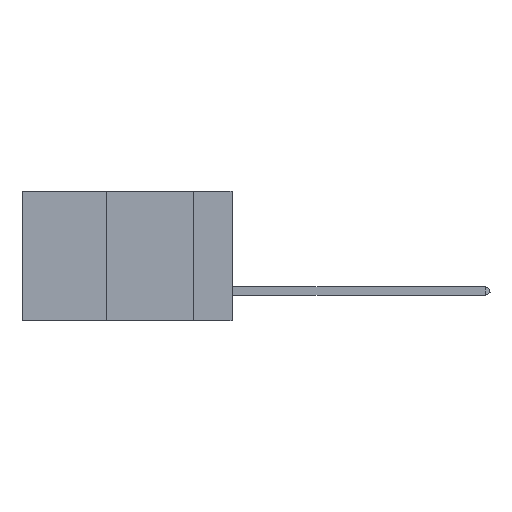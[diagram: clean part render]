
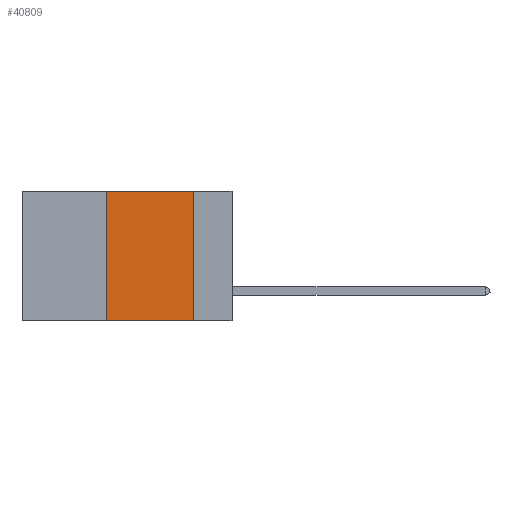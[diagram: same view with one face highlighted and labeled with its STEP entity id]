
A CAD part, left-side view. The second image highlights one B-rep face of the part: STEP entity #40809.
In plain terms, the highlighted planar face has unit normal (-1, 0, 0).
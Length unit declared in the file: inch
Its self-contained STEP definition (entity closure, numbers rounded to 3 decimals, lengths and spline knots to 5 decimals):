
#551 = DIRECTION ( 'NONE',  ( 0., -1., 0. ) ) ;
#1785 = VECTOR ( 'NONE', #551, 39.37008 ) ;
#2570 = EDGE_CURVE ( 'NONE', #17723, #35782, #29500, .T. ) ;
#2964 = VECTOR ( 'NONE', #40198, 39.37008 ) ;
#3206 = LINE ( 'NONE', #25588, #14075 ) ;
#4527 = ORIENTED_EDGE ( 'NONE', *, *, #42694, .F. ) ;
#5958 = FACE_OUTER_BOUND ( 'NONE', #35866, .T. ) ;
#7926 = PLANE ( 'NONE',  #23742 ) ;
#8074 = DIRECTION ( 'NONE',  ( 0., 0., -1. ) ) ;
#8186 = VECTOR ( 'NONE', #39829, 39.37008 ) ;
#10314 = CARTESIAN_POINT ( 'NONE',  ( 0., 0.11, -0.37 ) ) ;
#10552 = LINE ( 'NONE', #36775, #1785 ) ;
#14075 = VECTOR ( 'NONE', #31936, 39.37008 ) ;
#17723 = VERTEX_POINT ( 'NONE', #24574 ) ;
#19041 = LINE ( 'NONE', #20052, #2964 ) ;
#20052 = CARTESIAN_POINT ( 'NONE',  ( 0., 0.11, 0. ) ) ;
#20789 = DIRECTION ( 'NONE',  ( 1., 0., 0. ) ) ;
#21917 = EDGE_CURVE ( 'NONE', #35782, #30737, #10552, .T. ) ;
#21970 = VERTEX_POINT ( 'NONE', #10314 ) ;
#22845 = EDGE_CURVE ( 'NONE', #17723, #21970, #3206, .T. ) ;
#23742 = AXIS2_PLACEMENT_3D ( 'NONE', #24183, #20789, #8074 ) ;
#24183 = CARTESIAN_POINT ( 'NONE',  ( 0., 0.6, 0. ) ) ;
#24574 = CARTESIAN_POINT ( 'NONE',  ( 0., 0.36, -0.37 ) ) ;
#25588 = CARTESIAN_POINT ( 'NONE',  ( 0., 0.6, -0.37 ) ) ;
#26055 = CARTESIAN_POINT ( 'NONE',  ( 0., 0.11, 0. ) ) ;
#28347 = ORIENTED_EDGE ( 'NONE', *, *, #21917, .F. ) ;
#29495 = CARTESIAN_POINT ( 'NONE',  ( 0., 0.36, 0. ) ) ;
#29500 = LINE ( 'NONE', #29495, #8186 ) ;
#30737 = VERTEX_POINT ( 'NONE', #26055 ) ;
#31936 = DIRECTION ( 'NONE',  ( 0., -1., 0. ) ) ;
#35782 = VERTEX_POINT ( 'NONE', #38615 ) ;
#35866 = EDGE_LOOP ( 'NONE', ( #4527, #28347, #36657, #39334 ) ) ;
#36657 = ORIENTED_EDGE ( 'NONE', *, *, #2570, .F. ) ;
#36775 = CARTESIAN_POINT ( 'NONE',  ( 0., 0.6, 0. ) ) ;
#38615 = CARTESIAN_POINT ( 'NONE',  ( 0., 0.36, 0. ) ) ;
#39334 = ORIENTED_EDGE ( 'NONE', *, *, #22845, .T. ) ;
#39829 = DIRECTION ( 'NONE',  ( 0., 0., 1. ) ) ;
#40198 = DIRECTION ( 'NONE',  ( 0., 0., -1. ) ) ;
#40809 = ADVANCED_FACE ( 'NONE', ( #5958 ), #7926, .F. ) ;
#42694 = EDGE_CURVE ( 'NONE', #30737, #21970, #19041, .T. ) ;
